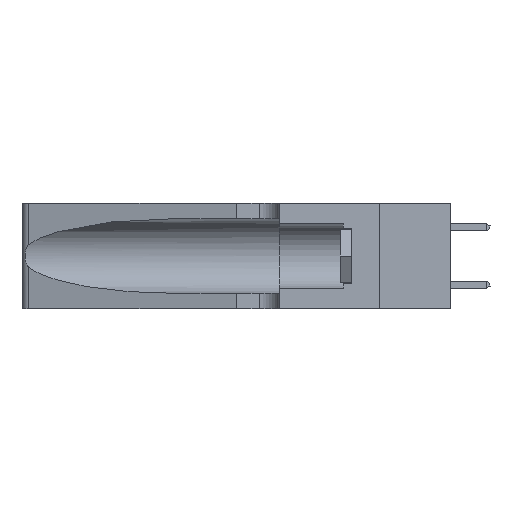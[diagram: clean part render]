
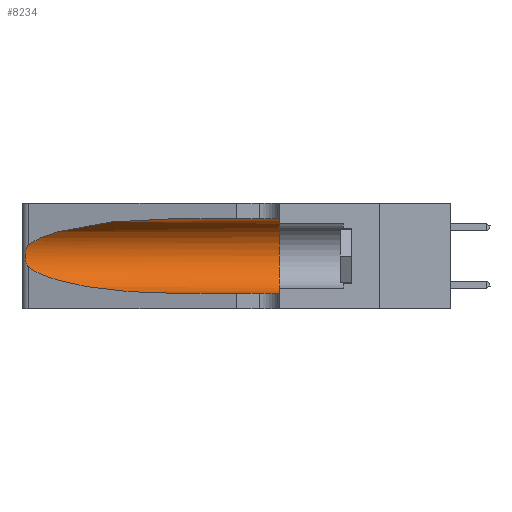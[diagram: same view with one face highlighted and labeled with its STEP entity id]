
A CAD part, left-side view. The second image highlights one B-rep face of the part: STEP entity #8234.
In plain terms, the highlighted cylindrical face has radius 3.308 mm (diameter 6.617 mm), a partial arc.
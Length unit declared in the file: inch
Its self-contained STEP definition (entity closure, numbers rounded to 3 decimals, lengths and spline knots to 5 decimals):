
#70 = ORIENTED_EDGE ( 'NONE', *, *, #22017, .F. ) ;
#590 = CARTESIAN_POINT ( 'NONE',  ( 0.1305, 0.72297, 0.05475 ) ) ;
#660 = CARTESIAN_POINT ( 'NONE',  ( 0.25487, 1.22718, 0.14631 ) ) ;
#678 = CARTESIAN_POINT ( 'NONE',  ( 0.2373, 1.15595, 0.08982 ) ) ;
#1089 =( BOUNDED_CURVE ( )  B_SPLINE_CURVE ( 3, ( #17063, #18749, #8642, #20494 ),
 .UNSPECIFIED., .F., .F. ) 
 B_SPLINE_CURVE_WITH_KNOTS ( ( 4, 4 ),
 ( 1.5708, 2.84003 ),
 .UNSPECIFIED. ) 
 CURVE ( )  GEOMETRIC_REPRESENTATION_ITEM ( )  RATIONAL_B_SPLINE_CURVE ( ( 1., 0.87, 0.87, 1. ) ) 
 REPRESENTATION_ITEM ( '' )  );
#1294 = CARTESIAN_POINT ( 'NONE',  ( 0.25487, 1.22718, 0.22369 ) ) ;
#1355 = CARTESIAN_POINT ( 'NONE',  ( 0.25787, 1.23484, 0.2124 ) ) ;
#1516 = EDGE_CURVE ( 'NONE', #5710, #5359, #15741, .T. ) ;
#1547 = EDGE_CURVE ( 'NONE', #3149, #7689, #2798, .T. ) ;
#2798 =( BOUNDED_CURVE ( )  B_SPLINE_CURVE ( 3, ( #660, #678, #18151, #590 ),
 .UNSPECIFIED., .F., .F. ) 
 B_SPLINE_CURVE_WITH_KNOTS ( ( 4, 4 ),
 ( 3.44316, 4.71239 ),
 .UNSPECIFIED. ) 
 CURVE ( )  GEOMETRIC_REPRESENTATION_ITEM ( )  RATIONAL_B_SPLINE_CURVE ( ( 1., 0.87, 0.87, 1. ) ) 
 REPRESENTATION_ITEM ( '' )  );
#3149 = VERTEX_POINT ( 'NONE', #16386 ) ;
#3158 = CARTESIAN_POINT ( 'NONE',  ( 0.26018, 1.23835, 0.19895 ) ) ;
#3687 = CARTESIAN_POINT ( 'NONE',  ( 0.1305, 1.61858, 0.05475 ) ) ;
#4109 = CARTESIAN_POINT ( 'NONE',  ( 0.1305, 0.72297, 0.31525 ) ) ;
#4130 = CARTESIAN_POINT ( 'NONE',  ( 0.1305, 0.35, 0.185 ) ) ;
#4219 = ORIENTED_EDGE ( 'NONE', *, *, #21852, .T. ) ;
#4642 = ORIENTED_EDGE ( 'NONE', *, *, #18383, .T. ) ;
#4885 = CARTESIAN_POINT ( 'NONE',  ( 0.26075, 1.23896, 0.178 ) ) ;
#5147 = B_SPLINE_CURVE_WITH_KNOTS ( 'NONE', 3,
 ( #1294, #20106, #11693, #1355, #13417, #3158, #15100, #4885, #16768, #6632, #18460, #8357, #20192, #10074 ),
 .UNSPECIFIED., .F., .F.,
 ( 4, 2, 2, 2, 2, 2, 4 ),
 ( 0., 0.00027, 0.00053, 0.00107, 0.0016, 0.00187, 0.00214 ),
 .UNSPECIFIED. ) ;
#5359 = VERTEX_POINT ( 'NONE', #10442 ) ;
#5662 = CARTESIAN_POINT ( 'NONE',  ( 0.1305, 0.35, 0.31525 ) ) ;
#5679 = CARTESIAN_POINT ( 'NONE',  ( 0.25487, 1.22718, 0.22369 ) ) ;
#5710 = VERTEX_POINT ( 'NONE', #5662 ) ;
#6132 = DIRECTION ( 'NONE',  ( 0., -1., 0. ) ) ;
#6632 = CARTESIAN_POINT ( 'NONE',  ( 0.25856, 1.23593, 0.16098 ) ) ;
#7523 = CARTESIAN_POINT ( 'NONE',  ( 0.1305, 1.61858, 0.185 ) ) ;
#7689 = VERTEX_POINT ( 'NONE', #14529 ) ;
#8185 = EDGE_LOOP ( 'NONE', ( #4642, #8601, #16197, #4219, #15313, #70 ) ) ;
#8234 = ADVANCED_FACE ( 'NONE', ( #8412 ), #16855, .F. ) ;
#8357 = CARTESIAN_POINT ( 'NONE',  ( 0.25639, 1.23186, 0.15144 ) ) ;
#8412 = FACE_OUTER_BOUND ( 'NONE', #8185, .T. ) ;
#8601 = ORIENTED_EDGE ( 'NONE', *, *, #18271, .T. ) ;
#8642 = CARTESIAN_POINT ( 'NONE',  ( 0.2373, 1.15595, 0.28018 ) ) ;
#10074 = CARTESIAN_POINT ( 'NONE',  ( 0.25487, 1.22718, 0.14631 ) ) ;
#10442 = CARTESIAN_POINT ( 'NONE',  ( 0.1305, 0.35, 0.05475 ) ) ;
#11275 = CARTESIAN_POINT ( 'NONE',  ( 0.1305, 1.61858, 0.31525 ) ) ;
#11693 = CARTESIAN_POINT ( 'NONE',  ( 0.25639, 1.23184, 0.21858 ) ) ;
#11909 = VECTOR ( 'NONE', #6132, 39.37008 ) ;
#13417 = CARTESIAN_POINT ( 'NONE',  ( 0.25854, 1.2359, 0.20912 ) ) ;
#14529 = CARTESIAN_POINT ( 'NONE',  ( 0.1305, 0.72297, 0.05475 ) ) ;
#15100 = CARTESIAN_POINT ( 'NONE',  ( 0.26075, 1.23896, 0.19203 ) ) ;
#15313 = ORIENTED_EDGE ( 'NONE', *, *, #1516, .F. ) ;
#15741 = CIRCLE ( 'NONE', #21918, 0.13025 ) ;
#15779 = VERTEX_POINT ( 'NONE', #5679 ) ;
#15887 = DIRECTION ( 'NONE',  ( 0., 0., -1. ) ) ;
#15971 = DIRECTION ( 'NONE',  ( 0., -1., 0. ) ) ;
#16197 = ORIENTED_EDGE ( 'NONE', *, *, #1547, .T. ) ;
#16386 = CARTESIAN_POINT ( 'NONE',  ( 0.25487, 1.22718, 0.14631 ) ) ;
#16651 = VECTOR ( 'NONE', #17289, 39.37008 ) ;
#16768 = CARTESIAN_POINT ( 'NONE',  ( 0.26017, 1.23833, 0.17102 ) ) ;
#16855 = CYLINDRICAL_SURFACE ( 'NONE', #17165, 0.13025 ) ;
#16988 = VERTEX_POINT ( 'NONE', #4109 ) ;
#17063 = CARTESIAN_POINT ( 'NONE',  ( 0.1305, 0.72297, 0.31525 ) ) ;
#17165 = AXIS2_PLACEMENT_3D ( 'NONE', #7523, #15971, #15887 ) ;
#17289 = DIRECTION ( 'NONE',  ( 0., -1., 0. ) ) ;
#18151 = CARTESIAN_POINT ( 'NONE',  ( 0.18966, 0.96281, 0.05475 ) ) ;
#18271 = EDGE_CURVE ( 'NONE', #15779, #3149, #5147, .T. ) ;
#18383 = EDGE_CURVE ( 'NONE', #16988, #15779, #1089, .T. ) ;
#18460 = CARTESIAN_POINT ( 'NONE',  ( 0.25789, 1.23486, 0.15765 ) ) ;
#18749 = CARTESIAN_POINT ( 'NONE',  ( 0.18966, 0.96281, 0.31525 ) ) ;
#19304 = DIRECTION ( 'NONE',  ( 0., 1., 0. ) ) ;
#19439 = DIRECTION ( 'NONE',  ( 0., 0., 1. ) ) ;
#20106 = CARTESIAN_POINT ( 'NONE',  ( 0.25555, 1.22994, 0.2215 ) ) ;
#20107 = LINE ( 'NONE', #3687, #16651 ) ;
#20192 = CARTESIAN_POINT ( 'NONE',  ( 0.25555, 1.22993, 0.14849 ) ) ;
#20494 = CARTESIAN_POINT ( 'NONE',  ( 0.25487, 1.22718, 0.22369 ) ) ;
#20898 = LINE ( 'NONE', #11275, #11909 ) ;
#21852 = EDGE_CURVE ( 'NONE', #7689, #5359, #20107, .T. ) ;
#21918 = AXIS2_PLACEMENT_3D ( 'NONE', #4130, #19304, #19439 ) ;
#22017 = EDGE_CURVE ( 'NONE', #16988, #5710, #20898, .T. ) ;
